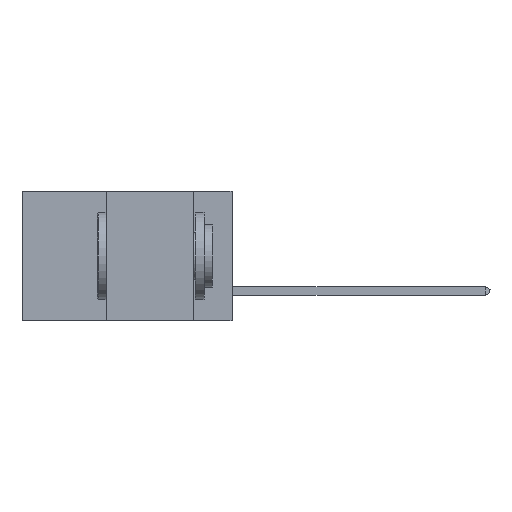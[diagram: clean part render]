
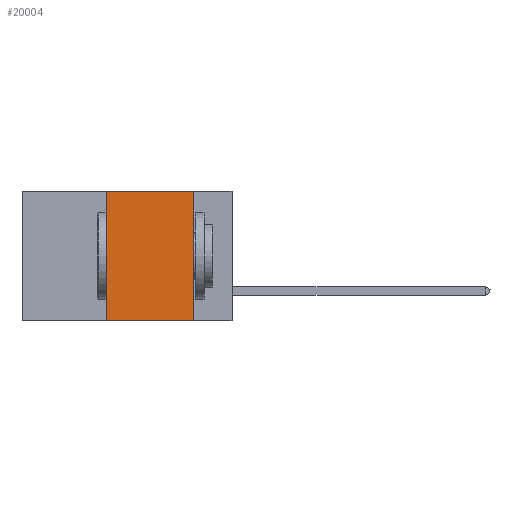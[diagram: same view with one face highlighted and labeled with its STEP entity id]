
A CAD part, left-side view. The second image highlights one B-rep face of the part: STEP entity #20004.
In plain terms, the highlighted planar face has unit normal (-1, 0, 0).
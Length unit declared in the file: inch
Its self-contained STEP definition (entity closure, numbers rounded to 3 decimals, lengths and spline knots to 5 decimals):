
#1097 = VECTOR ( 'NONE', #19253, 39.37008 ) ;
#2759 = AXIS2_PLACEMENT_3D ( 'NONE', #29280, #14765, #17686 ) ;
#3282 = VERTEX_POINT ( 'NONE', #4017 ) ;
#4017 = CARTESIAN_POINT ( 'NONE',  ( 0., 0.36, 0. ) ) ;
#5079 = EDGE_CURVE ( 'NONE', #3282, #30385, #16631, .T. ) ;
#5349 = VECTOR ( 'NONE', #11096, 39.37008 ) ;
#5912 = ORIENTED_EDGE ( 'NONE', *, *, #22612, .F. ) ;
#7853 = CARTESIAN_POINT ( 'NONE',  ( 0., 0.11, 0. ) ) ;
#8055 = CARTESIAN_POINT ( 'NONE',  ( 0., 0.11, 0. ) ) ;
#8674 = PLANE ( 'NONE',  #2759 ) ;
#10099 = ORIENTED_EDGE ( 'NONE', *, *, #5079, .F. ) ;
#11096 = DIRECTION ( 'NONE',  ( 0., -1., 0. ) ) ;
#11395 = EDGE_CURVE ( 'NONE', #16262, #27536, #11686, .T. ) ;
#11686 = LINE ( 'NONE', #26275, #5349 ) ;
#14182 = CARTESIAN_POINT ( 'NONE',  ( 0., 0.11, -0.37 ) ) ;
#14765 = DIRECTION ( 'NONE',  ( 1., 0., 0. ) ) ;
#16262 = VERTEX_POINT ( 'NONE', #25382 ) ;
#16631 = LINE ( 'NONE', #33914, #1097 ) ;
#17686 = DIRECTION ( 'NONE',  ( 0., 0., -1. ) ) ;
#19051 = ORIENTED_EDGE ( 'NONE', *, *, #11395, .T. ) ;
#19253 = DIRECTION ( 'NONE',  ( 0., -1., 0. ) ) ;
#19529 = DIRECTION ( 'NONE',  ( 0., 0., -1. ) ) ;
#19850 = EDGE_LOOP ( 'NONE', ( #33296, #10099, #5912, #19051 ) ) ;
#20004 = ADVANCED_FACE ( 'NONE', ( #21887 ), #8674, .F. ) ;
#20143 = LINE ( 'NONE', #8055, #35724 ) ;
#20225 = VECTOR ( 'NONE', #22676, 39.37008 ) ;
#21887 = FACE_OUTER_BOUND ( 'NONE', #19850, .T. ) ;
#22612 = EDGE_CURVE ( 'NONE', #16262, #3282, #27097, .T. ) ;
#22676 = DIRECTION ( 'NONE',  ( 0., 0., 1. ) ) ;
#25382 = CARTESIAN_POINT ( 'NONE',  ( 0., 0.36, -0.37 ) ) ;
#25779 = CARTESIAN_POINT ( 'NONE',  ( 0., 0.36, 0. ) ) ;
#26275 = CARTESIAN_POINT ( 'NONE',  ( 0., 0.6, -0.37 ) ) ;
#27097 = LINE ( 'NONE', #25779, #20225 ) ;
#27536 = VERTEX_POINT ( 'NONE', #14182 ) ;
#29280 = CARTESIAN_POINT ( 'NONE',  ( 0., 0.6, 0. ) ) ;
#29939 = EDGE_CURVE ( 'NONE', #30385, #27536, #20143, .T. ) ;
#30385 = VERTEX_POINT ( 'NONE', #7853 ) ;
#33296 = ORIENTED_EDGE ( 'NONE', *, *, #29939, .F. ) ;
#33914 = CARTESIAN_POINT ( 'NONE',  ( 0., 0.6, 0. ) ) ;
#35724 = VECTOR ( 'NONE', #19529, 39.37008 ) ;
